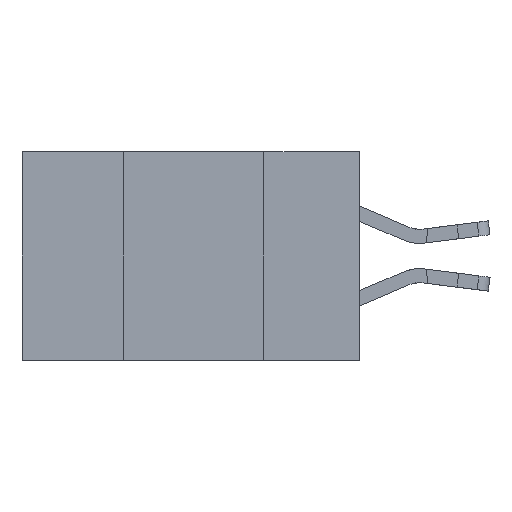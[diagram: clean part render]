
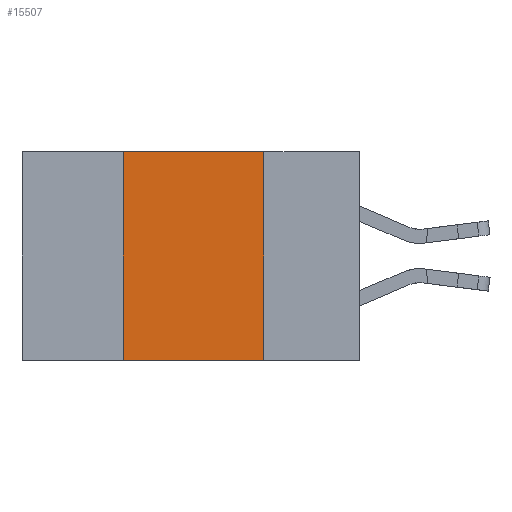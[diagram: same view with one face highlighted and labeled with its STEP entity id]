
A CAD part, left-side view. The second image highlights one B-rep face of the part: STEP entity #15507.
In plain terms, the highlighted planar face has unit normal (-1, 0, 0).
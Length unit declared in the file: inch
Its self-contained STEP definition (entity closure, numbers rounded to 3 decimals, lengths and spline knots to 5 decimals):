
#322 = EDGE_CURVE ( 'NONE', #10107, #10596, #5677, .T. ) ;
#732 = LINE ( 'NONE', #10738, #5391 ) ;
#1279 = AXIS2_PLACEMENT_3D ( 'NONE', #9858, #11388, #2191 ) ;
#1332 = FACE_OUTER_BOUND ( 'NONE', #2465, .T. ) ;
#1437 = ORIENTED_EDGE ( 'NONE', *, *, #322, .F. ) ;
#2191 = DIRECTION ( 'NONE',  ( 0., 0., -1. ) ) ;
#2465 = EDGE_LOOP ( 'NONE', ( #1437, #3567, #7953, #14961 ) ) ;
#3199 = DIRECTION ( 'NONE',  ( 0., 0., -1. ) ) ;
#3567 = ORIENTED_EDGE ( 'NONE', *, *, #11801, .F. ) ;
#3745 = CARTESIAN_POINT ( 'NONE',  ( 0., 0.17, 0. ) ) ;
#4082 = VERTEX_POINT ( 'NONE', #19364 ) ;
#5391 = VECTOR ( 'NONE', #6220, 39.37008 ) ;
#5677 = LINE ( 'NONE', #3745, #17296 ) ;
#6220 = DIRECTION ( 'NONE',  ( 0., -1., 0. ) ) ;
#6698 = DIRECTION ( 'NONE',  ( 0., -1., 0. ) ) ;
#7171 = VERTEX_POINT ( 'NONE', #8012 ) ;
#7660 = CARTESIAN_POINT ( 'NONE',  ( 0., 0.17, -0.37 ) ) ;
#7953 = ORIENTED_EDGE ( 'NONE', *, *, #11167, .F. ) ;
#8012 = CARTESIAN_POINT ( 'NONE',  ( 0., 0.42, -0.37 ) ) ;
#9135 = EDGE_CURVE ( 'NONE', #7171, #10596, #16197, .T. ) ;
#9603 = CARTESIAN_POINT ( 'NONE',  ( 0., 0.17, 0. ) ) ;
#9858 = CARTESIAN_POINT ( 'NONE',  ( 0., 0.6, 0. ) ) ;
#10107 = VERTEX_POINT ( 'NONE', #9603 ) ;
#10596 = VERTEX_POINT ( 'NONE', #7660 ) ;
#10738 = CARTESIAN_POINT ( 'NONE',  ( 0., 0.6, 0. ) ) ;
#11167 = EDGE_CURVE ( 'NONE', #7171, #4082, #15414, .T. ) ;
#11388 = DIRECTION ( 'NONE',  ( 1., 0., 0. ) ) ;
#11801 = EDGE_CURVE ( 'NONE', #4082, #10107, #732, .T. ) ;
#14961 = ORIENTED_EDGE ( 'NONE', *, *, #9135, .T. ) ;
#15071 = CARTESIAN_POINT ( 'NONE',  ( 0., 0.42, 0. ) ) ;
#15414 = LINE ( 'NONE', #15071, #18936 ) ;
#15507 = ADVANCED_FACE ( 'NONE', ( #1332 ), #18914, .F. ) ;
#16197 = LINE ( 'NONE', #17275, #19715 ) ;
#16581 = DIRECTION ( 'NONE',  ( 0., 0., 1. ) ) ;
#17275 = CARTESIAN_POINT ( 'NONE',  ( 0., 0.6, -0.37 ) ) ;
#17296 = VECTOR ( 'NONE', #3199, 39.37008 ) ;
#18914 = PLANE ( 'NONE',  #1279 ) ;
#18936 = VECTOR ( 'NONE', #16581, 39.37008 ) ;
#19364 = CARTESIAN_POINT ( 'NONE',  ( 0., 0.42, 0. ) ) ;
#19715 = VECTOR ( 'NONE', #6698, 39.37008 ) ;
